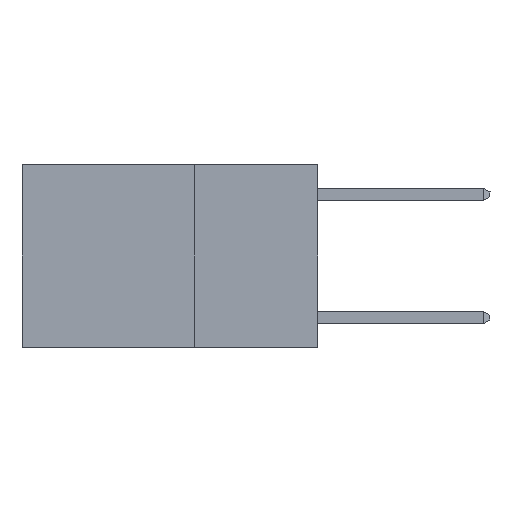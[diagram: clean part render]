
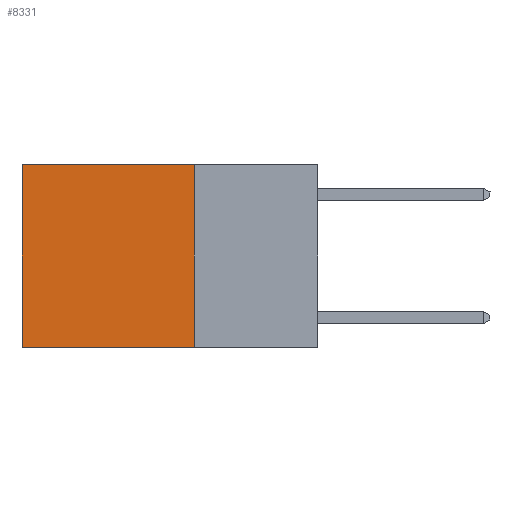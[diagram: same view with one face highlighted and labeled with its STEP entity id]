
A CAD part, left-side view. The second image highlights one B-rep face of the part: STEP entity #8331.
In plain terms, the highlighted planar face has unit normal (-1, 0, 0).
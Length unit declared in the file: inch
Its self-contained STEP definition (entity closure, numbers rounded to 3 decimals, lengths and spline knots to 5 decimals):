
#360 = DIRECTION ( 'NONE',  ( 1., 0., 0. ) ) ;
#701 = DIRECTION ( 'NONE',  ( 0., 1., 0. ) ) ;
#708 = VERTEX_POINT ( 'NONE', #4157 ) ;
#1190 = FACE_OUTER_BOUND ( 'NONE', #12020, .T. ) ;
#1735 = VECTOR ( 'NONE', #701, 39.37008 ) ;
#1739 = LINE ( 'NONE', #5810, #13229 ) ;
#4157 = CARTESIAN_POINT ( 'NONE',  ( 0.2625, 0.6, -0.37 ) ) ;
#4944 = VERTEX_POINT ( 'NONE', #12478 ) ;
#5544 = ORIENTED_EDGE ( 'NONE', *, *, #6850, .T. ) ;
#5810 = CARTESIAN_POINT ( 'NONE',  ( 0.2625, 0.25, 0. ) ) ;
#5989 = DIRECTION ( 'NONE',  ( 0., 0., -1. ) ) ;
#6850 = EDGE_CURVE ( 'NONE', #4944, #708, #16435, .T. ) ;
#7888 = VERTEX_POINT ( 'NONE', #14887 ) ;
#8101 = CARTESIAN_POINT ( 'NONE',  ( 0.2625, 0.25, 0. ) ) ;
#8331 = ADVANCED_FACE ( 'NONE', ( #1190 ), #13153, .F. ) ;
#9340 = EDGE_CURVE ( 'NONE', #7888, #4944, #13982, .T. ) ;
#9394 = DIRECTION ( 'NONE',  ( 0., 0., -1. ) ) ;
#9684 = AXIS2_PLACEMENT_3D ( 'NONE', #8101, #360, #9394 ) ;
#9884 = CARTESIAN_POINT ( 'NONE',  ( 0.2625, 0.6, 0. ) ) ;
#9912 = EDGE_CURVE ( 'NONE', #11375, #708, #11980, .T. ) ;
#10725 = ORIENTED_EDGE ( 'NONE', *, *, #9340, .T. ) ;
#10989 = CARTESIAN_POINT ( 'NONE',  ( 0.2625, 0.25, -0.37 ) ) ;
#11375 = VERTEX_POINT ( 'NONE', #15983 ) ;
#11980 = LINE ( 'NONE', #10989, #1735 ) ;
#12020 = EDGE_LOOP ( 'NONE', ( #5544, #12347, #15789, #10725 ) ) ;
#12199 = DIRECTION ( 'NONE',  ( 0., 0., -1. ) ) ;
#12347 = ORIENTED_EDGE ( 'NONE', *, *, #9912, .F. ) ;
#12478 = CARTESIAN_POINT ( 'NONE',  ( 0.2625, 0.6, 0. ) ) ;
#13153 = PLANE ( 'NONE',  #9684 ) ;
#13180 = VECTOR ( 'NONE', #13739, 39.37008 ) ;
#13229 = VECTOR ( 'NONE', #12199, 39.37008 ) ;
#13739 = DIRECTION ( 'NONE',  ( 0., 1., 0. ) ) ;
#13982 = LINE ( 'NONE', #16273, #13180 ) ;
#14887 = CARTESIAN_POINT ( 'NONE',  ( 0.2625, 0.25, 0. ) ) ;
#15789 = ORIENTED_EDGE ( 'NONE', *, *, #16017, .F. ) ;
#15983 = CARTESIAN_POINT ( 'NONE',  ( 0.2625, 0.25, -0.37 ) ) ;
#16016 = VECTOR ( 'NONE', #5989, 39.37008 ) ;
#16017 = EDGE_CURVE ( 'NONE', #7888, #11375, #1739, .T. ) ;
#16273 = CARTESIAN_POINT ( 'NONE',  ( 0.2625, 0.25, 0. ) ) ;
#16435 = LINE ( 'NONE', #9884, #16016 ) ;
